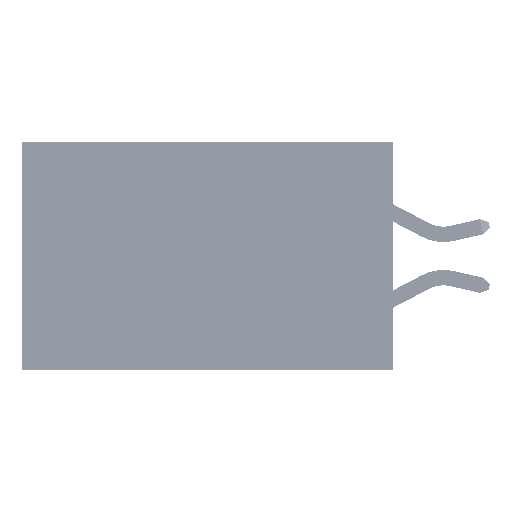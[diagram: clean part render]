
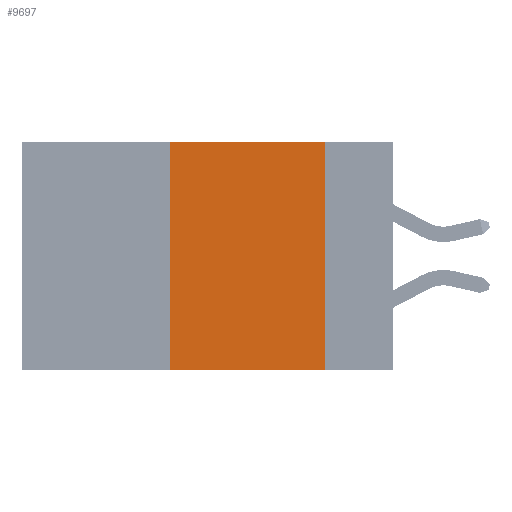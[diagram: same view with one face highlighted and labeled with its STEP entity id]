
A CAD part, left-side view. The second image highlights one B-rep face of the part: STEP entity #9697.
In plain terms, the highlighted planar face has unit normal (-1, 0, 0).
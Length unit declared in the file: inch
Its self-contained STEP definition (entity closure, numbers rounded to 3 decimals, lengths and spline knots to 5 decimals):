
#2054 = VERTEX_POINT ( 'NONE', #29672 ) ;
#2530 = CARTESIAN_POINT ( 'NONE',  ( 0., 0.36, -0.37 ) ) ;
#2949 = VERTEX_POINT ( 'NONE', #8637 ) ;
#3986 = DIRECTION ( 'NONE',  ( 0., 0., -1. ) ) ;
#4086 = DIRECTION ( 'NONE',  ( 0., -1., 0. ) ) ;
#4238 = FACE_OUTER_BOUND ( 'NONE', #45048, .T. ) ;
#7484 = VECTOR ( 'NONE', #4086, 39.37008 ) ;
#8637 = CARTESIAN_POINT ( 'NONE',  ( 0., 0.36, 0. ) ) ;
#9697 = ADVANCED_FACE ( 'NONE', ( #4238 ), #22219, .F. ) ;
#11220 = LINE ( 'NONE', #36311, #7484 ) ;
#11560 = CARTESIAN_POINT ( 'NONE',  ( 0., 0.6, 0. ) ) ;
#12609 = VECTOR ( 'NONE', #12755, 39.37008 ) ;
#12755 = DIRECTION ( 'NONE',  ( 0., -1., 0. ) ) ;
#13312 = CARTESIAN_POINT ( 'NONE',  ( 0., 0.11, -0.37 ) ) ;
#14067 = EDGE_CURVE ( 'NONE', #2054, #17461, #18764, .T. ) ;
#15218 = DIRECTION ( 'NONE',  ( 0., 0., 1. ) ) ;
#15918 = EDGE_CURVE ( 'NONE', #2949, #2054, #11220, .T. ) ;
#16109 = DIRECTION ( 'NONE',  ( 0., 0., -1. ) ) ;
#17115 = VECTOR ( 'NONE', #16109, 39.37008 ) ;
#17461 = VERTEX_POINT ( 'NONE', #13312 ) ;
#18764 = LINE ( 'NONE', #37217, #17115 ) ;
#18792 = LINE ( 'NONE', #33255, #45804 ) ;
#20959 = VERTEX_POINT ( 'NONE', #2530 ) ;
#21469 = AXIS2_PLACEMENT_3D ( 'NONE', #11560, #37132, #3986 ) ;
#22219 = PLANE ( 'NONE',  #21469 ) ;
#24036 = ORIENTED_EDGE ( 'NONE', *, *, #14067, .F. ) ;
#27699 = ORIENTED_EDGE ( 'NONE', *, *, #42521, .T. ) ;
#29672 = CARTESIAN_POINT ( 'NONE',  ( 0., 0.11, 0. ) ) ;
#30503 = EDGE_CURVE ( 'NONE', #20959, #2949, #18792, .T. ) ;
#33255 = CARTESIAN_POINT ( 'NONE',  ( 0., 0.36, 0. ) ) ;
#34766 = LINE ( 'NONE', #45192, #12609 ) ;
#36311 = CARTESIAN_POINT ( 'NONE',  ( 0., 0.6, 0. ) ) ;
#37132 = DIRECTION ( 'NONE',  ( 1., 0., 0. ) ) ;
#37217 = CARTESIAN_POINT ( 'NONE',  ( 0., 0.11, 0. ) ) ;
#39492 = ORIENTED_EDGE ( 'NONE', *, *, #30503, .F. ) ;
#42521 = EDGE_CURVE ( 'NONE', #20959, #17461, #34766, .T. ) ;
#43824 = ORIENTED_EDGE ( 'NONE', *, *, #15918, .F. ) ;
#45048 = EDGE_LOOP ( 'NONE', ( #24036, #43824, #39492, #27699 ) ) ;
#45192 = CARTESIAN_POINT ( 'NONE',  ( 0., 0.6, -0.37 ) ) ;
#45804 = VECTOR ( 'NONE', #15218, 39.37008 ) ;
